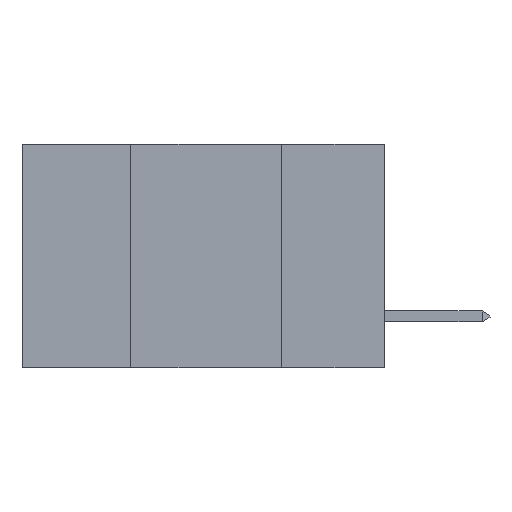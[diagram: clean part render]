
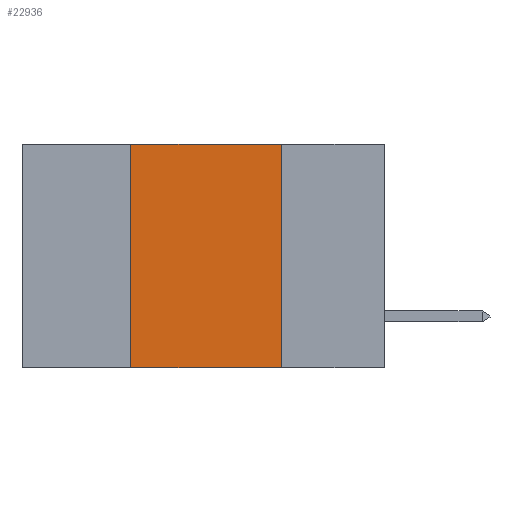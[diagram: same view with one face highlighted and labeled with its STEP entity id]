
A CAD part, left-side view. The second image highlights one B-rep face of the part: STEP entity #22936.
In plain terms, the highlighted planar face has unit normal (-1, 0, 0).
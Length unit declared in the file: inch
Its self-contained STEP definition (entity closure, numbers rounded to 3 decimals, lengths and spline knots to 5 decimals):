
#382 = VECTOR ( 'NONE', #7075, 39.37008 ) ;
#1070 = LINE ( 'NONE', #24226, #25092 ) ;
#1331 = LINE ( 'NONE', #4050, #382 ) ;
#1620 = CARTESIAN_POINT ( 'NONE',  ( 0., 0.17, 0. ) ) ;
#2240 = EDGE_CURVE ( 'NONE', #29184, #2606, #31473, .T. ) ;
#2606 = VERTEX_POINT ( 'NONE', #27609 ) ;
#3190 = DIRECTION ( 'NONE',  ( 0., -1., 0. ) ) ;
#3574 = FACE_OUTER_BOUND ( 'NONE', #6127, .T. ) ;
#4050 = CARTESIAN_POINT ( 'NONE',  ( 0., 0.6, 0. ) ) ;
#4350 = DIRECTION ( 'NONE',  ( 0., 0., -1. ) ) ;
#4363 = AXIS2_PLACEMENT_3D ( 'NONE', #13376, #22396, #4350 ) ;
#4789 = DIRECTION ( 'NONE',  ( 0., 0., -1. ) ) ;
#6127 = EDGE_LOOP ( 'NONE', ( #6964, #6520, #24406, #8865 ) ) ;
#6520 = ORIENTED_EDGE ( 'NONE', *, *, #21110, .F. ) ;
#6964 = ORIENTED_EDGE ( 'NONE', *, *, #8800, .F. ) ;
#7075 = DIRECTION ( 'NONE',  ( 0., -1., 0. ) ) ;
#7373 = CARTESIAN_POINT ( 'NONE',  ( 0., 0.42, -0.37 ) ) ;
#8800 = EDGE_CURVE ( 'NONE', #38042, #10513, #34682, .T. ) ;
#8865 = ORIENTED_EDGE ( 'NONE', *, *, #24651, .T. ) ;
#10513 = VERTEX_POINT ( 'NONE', #22353 ) ;
#13376 = CARTESIAN_POINT ( 'NONE',  ( 0., 0.6, 0. ) ) ;
#21110 = EDGE_CURVE ( 'NONE', #2606, #38042, #1331, .T. ) ;
#22353 = CARTESIAN_POINT ( 'NONE',  ( 0., 0.17, -0.37 ) ) ;
#22396 = DIRECTION ( 'NONE',  ( 1., 0., 0. ) ) ;
#22754 = VECTOR ( 'NONE', #34681, 39.37008 ) ;
#22936 = ADVANCED_FACE ( 'NONE', ( #3574 ), #37027, .F. ) ;
#24226 = CARTESIAN_POINT ( 'NONE',  ( 0., 0.6, -0.37 ) ) ;
#24406 = ORIENTED_EDGE ( 'NONE', *, *, #2240, .F. ) ;
#24651 = EDGE_CURVE ( 'NONE', #29184, #10513, #1070, .T. ) ;
#25092 = VECTOR ( 'NONE', #3190, 39.37008 ) ;
#25835 = CARTESIAN_POINT ( 'NONE',  ( 0., 0.42, 0. ) ) ;
#27609 = CARTESIAN_POINT ( 'NONE',  ( 0., 0.42, 0. ) ) ;
#27800 = VECTOR ( 'NONE', #4789, 39.37008 ) ;
#29184 = VERTEX_POINT ( 'NONE', #7373 ) ;
#31473 = LINE ( 'NONE', #25835, #22754 ) ;
#34681 = DIRECTION ( 'NONE',  ( 0., 0., 1. ) ) ;
#34682 = LINE ( 'NONE', #1620, #27800 ) ;
#37027 = PLANE ( 'NONE',  #4363 ) ;
#38042 = VERTEX_POINT ( 'NONE', #38374 ) ;
#38374 = CARTESIAN_POINT ( 'NONE',  ( 0., 0.17, 0. ) ) ;
